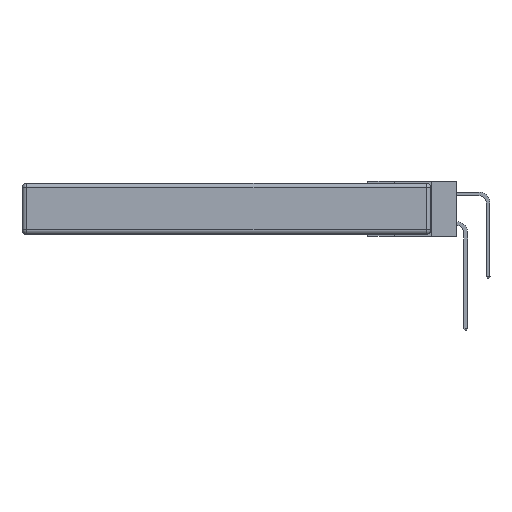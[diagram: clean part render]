
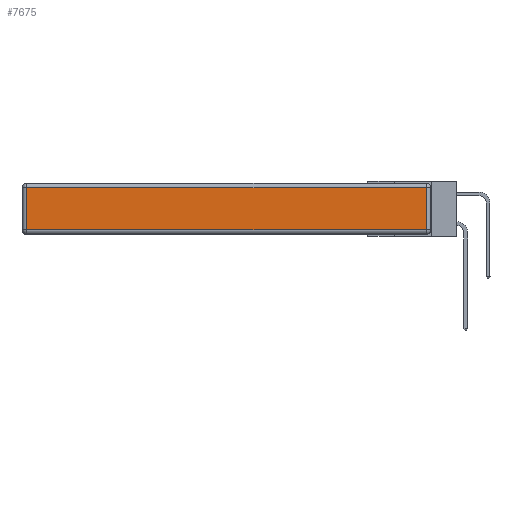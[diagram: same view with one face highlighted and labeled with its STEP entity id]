
A CAD part, left-side view. The second image highlights one B-rep face of the part: STEP entity #7675.
In plain terms, the highlighted planar face has unit normal (-1, 0, 0).
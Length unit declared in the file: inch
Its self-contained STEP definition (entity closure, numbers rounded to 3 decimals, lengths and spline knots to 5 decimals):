
#1852 = VERTEX_POINT ( 'NONE', #24069 ) ;
#2195 = PLANE ( 'NONE',  #10571 ) ;
#2466 = DIRECTION ( 'NONE',  ( 0., 0., -1. ) ) ;
#4228 = DIRECTION ( 'NONE',  ( 0., 0., 1. ) ) ;
#4244 = VECTOR ( 'NONE', #14554, 39.37008 ) ;
#4846 = CARTESIAN_POINT ( 'NONE',  ( 0., 0.03, -0.313 ) ) ;
#5046 = VERTEX_POINT ( 'NONE', #12049 ) ;
#5717 = EDGE_CURVE ( 'NONE', #1852, #5046, #24238, .T. ) ;
#7475 = VERTEX_POINT ( 'NONE', #4846 ) ;
#7675 = ADVANCED_FACE ( 'NONE', ( #16187 ), #2195, .T. ) ;
#9117 = CARTESIAN_POINT ( 'NONE',  ( 0., 0.03, -0.343 ) ) ;
#9268 = ORIENTED_EDGE ( 'NONE', *, *, #12671, .T. ) ;
#9343 = CARTESIAN_POINT ( 'NONE',  ( 0., 2.75, -0.03 ) ) ;
#9706 = EDGE_CURVE ( 'NONE', #10540, #7475, #19351, .T. ) ;
#9868 = DIRECTION ( 'NONE',  ( -1., 0., 0. ) ) ;
#10540 = VERTEX_POINT ( 'NONE', #10980 ) ;
#10571 = AXIS2_PLACEMENT_3D ( 'NONE', #11516, #9868, #4228 ) ;
#10909 = EDGE_CURVE ( 'NONE', #5046, #10540, #16658, .T. ) ;
#10980 = CARTESIAN_POINT ( 'NONE',  ( 0., 2.72, -0.313 ) ) ;
#11137 = ORIENTED_EDGE ( 'NONE', *, *, #5717, .T. ) ;
#11516 = CARTESIAN_POINT ( 'NONE',  ( 0., 0., -0.343 ) ) ;
#11866 = CARTESIAN_POINT ( 'NONE',  ( 0., 2.72, -0.343 ) ) ;
#12049 = CARTESIAN_POINT ( 'NONE',  ( 0., 2.72, -0.03 ) ) ;
#12169 = LINE ( 'NONE', #9117, #4244 ) ;
#12671 = EDGE_CURVE ( 'NONE', #7475, #1852, #12169, .T. ) ;
#14554 = DIRECTION ( 'NONE',  ( 0., 0., 1. ) ) ;
#15204 = ORIENTED_EDGE ( 'NONE', *, *, #9706, .T. ) ;
#16065 = VECTOR ( 'NONE', #2466, 39.37008 ) ;
#16127 = VECTOR ( 'NONE', #18880, 39.37008 ) ;
#16187 = FACE_OUTER_BOUND ( 'NONE', #24035, .T. ) ;
#16658 = LINE ( 'NONE', #11866, #16065 ) ;
#16909 = DIRECTION ( 'NONE',  ( 0., 1., 0. ) ) ;
#18880 = DIRECTION ( 'NONE',  ( 0., -1., 0. ) ) ;
#18957 = CARTESIAN_POINT ( 'NONE',  ( 0., 0., -0.313 ) ) ;
#19279 = VECTOR ( 'NONE', #16909, 39.37008 ) ;
#19351 = LINE ( 'NONE', #18957, #16127 ) ;
#24035 = EDGE_LOOP ( 'NONE', ( #15204, #9268, #11137, #24240 ) ) ;
#24069 = CARTESIAN_POINT ( 'NONE',  ( 0., 0.03, -0.03 ) ) ;
#24238 = LINE ( 'NONE', #9343, #19279 ) ;
#24240 = ORIENTED_EDGE ( 'NONE', *, *, #10909, .T. ) ;
